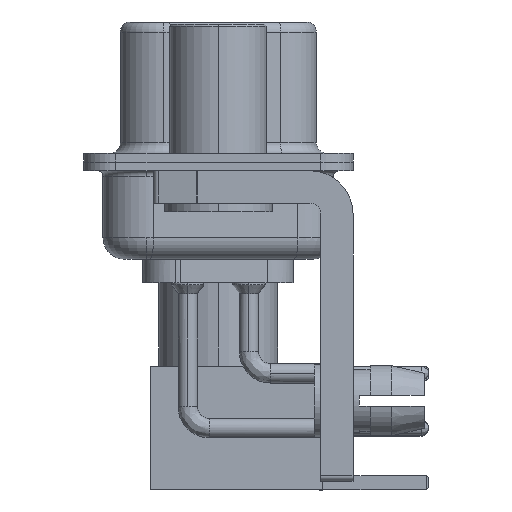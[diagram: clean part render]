
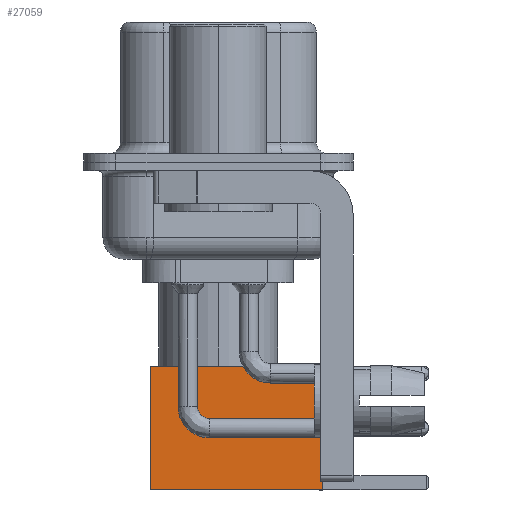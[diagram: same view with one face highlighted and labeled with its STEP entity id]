
A CAD part, left-side view. The second image highlights one B-rep face of the part: STEP entity #27059.
In plain terms, the highlighted face is planar.
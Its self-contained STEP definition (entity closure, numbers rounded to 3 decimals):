
#390 = DIRECTION ( 'NONE',  ( 0., 1., 0. ) ) ;
#1041 = VECTOR ( 'NONE', #10049, 1000. ) ;
#1836 = DIRECTION ( 'NONE',  ( -1., 0., 0. ) ) ;
#2215 = CARTESIAN_POINT ( 'NONE',  ( 2.875, 2.875, 0. ) ) ;
#3415 = VERTEX_POINT ( 'NONE', #22472 ) ;
#3417 = EDGE_CURVE ( 'NONE', #4890, #3415, #28060, .T. ) ;
#4269 = CARTESIAN_POINT ( 'NONE',  ( 0., 2.875, 8. ) ) ;
#4890 = VERTEX_POINT ( 'NONE', #17253 ) ;
#4939 = DIRECTION ( 'NONE',  ( 0., 0., 1. ) ) ;
#5094 = CARTESIAN_POINT ( 'NONE',  ( 2.875, 2.875, 0. ) ) ;
#6007 = EDGE_LOOP ( 'NONE', ( #28109, #29818, #20005, #24418 ) ) ;
#10049 = DIRECTION ( 'NONE',  ( 0., 0., -1. ) ) ;
#10161 = PLANE ( 'NONE',  #28975 ) ;
#11946 = LINE ( 'NONE', #24977, #18146 ) ;
#17164 = CARTESIAN_POINT ( 'NONE',  ( -2.875, 2.875, 0. ) ) ;
#17253 = CARTESIAN_POINT ( 'NONE',  ( 2.875, 2.875, 8. ) ) ;
#17470 = CARTESIAN_POINT ( 'NONE',  ( -2.875, 2.875, 0. ) ) ;
#18146 = VECTOR ( 'NONE', #1836, 1000. ) ;
#19982 = VECTOR ( 'NONE', #24851, 1000. ) ;
#20005 = ORIENTED_EDGE ( 'NONE', *, *, #29131, .F. ) ;
#20697 = VERTEX_POINT ( 'NONE', #17470 ) ;
#22472 = CARTESIAN_POINT ( 'NONE',  ( 2.875, 2.875, 0. ) ) ;
#22676 = DIRECTION ( 'NONE',  ( -1., 0., 0. ) ) ;
#23766 = VERTEX_POINT ( 'NONE', #32396 ) ;
#24418 = ORIENTED_EDGE ( 'NONE', *, *, #31359, .F. ) ;
#24851 = DIRECTION ( 'NONE',  ( 0., 0., -1. ) ) ;
#24977 = CARTESIAN_POINT ( 'NONE',  ( 0., 2.875, 0. ) ) ;
#27059 = ADVANCED_FACE ( 'NONE', ( #33345 ), #10161, .T. ) ;
#27425 = LINE ( 'NONE', #4269, #29539 ) ;
#27498 = LINE ( 'NONE', #17164, #1041 ) ;
#28060 = LINE ( 'NONE', #2215, #19982 ) ;
#28109 = ORIENTED_EDGE ( 'NONE', *, *, #3417, .T. ) ;
#28975 = AXIS2_PLACEMENT_3D ( 'NONE', #5094, #390, #4939 ) ;
#29131 = EDGE_CURVE ( 'NONE', #23766, #20697, #27498, .T. ) ;
#29539 = VECTOR ( 'NONE', #22676, 1000. ) ;
#29818 = ORIENTED_EDGE ( 'NONE', *, *, #32224, .T. ) ;
#31359 = EDGE_CURVE ( 'NONE', #4890, #23766, #27425, .T. ) ;
#32224 = EDGE_CURVE ( 'NONE', #3415, #20697, #11946, .T. ) ;
#32396 = CARTESIAN_POINT ( 'NONE',  ( -2.875, 2.875, 8. ) ) ;
#33345 = FACE_OUTER_BOUND ( 'NONE', #6007, .T. ) ;
